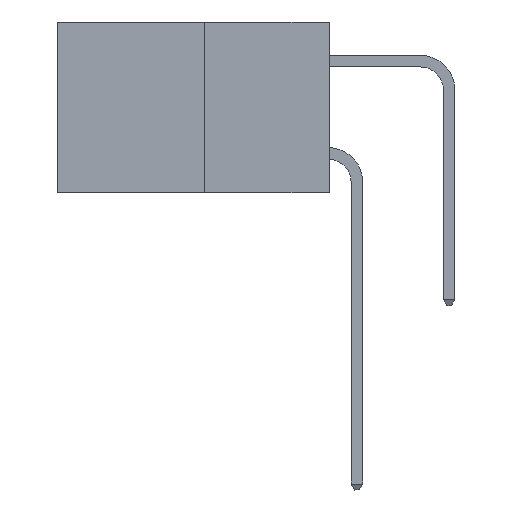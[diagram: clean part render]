
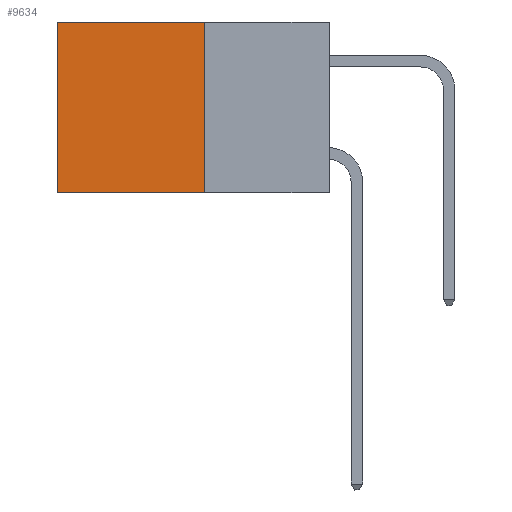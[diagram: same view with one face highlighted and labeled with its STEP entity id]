
A CAD part, left-side view. The second image highlights one B-rep face of the part: STEP entity #9634.
In plain terms, the highlighted planar face has unit normal (-1, 0, 0).
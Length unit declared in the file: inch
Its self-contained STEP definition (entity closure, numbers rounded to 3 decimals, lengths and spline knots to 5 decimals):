
#104 = DIRECTION ( 'NONE',  ( 0., 0., -1. ) ) ;
#999 = VECTOR ( 'NONE', #104, 39.37008 ) ;
#2378 = LINE ( 'NONE', #14865, #7768 ) ;
#2826 = DIRECTION ( 'NONE',  ( 0., 1., 0. ) ) ;
#3563 = VERTEX_POINT ( 'NONE', #7090 ) ;
#3830 = LINE ( 'NONE', #17312, #13896 ) ;
#3854 = DIRECTION ( 'NONE',  ( 1., 0., 0. ) ) ;
#4019 = AXIS2_PLACEMENT_3D ( 'NONE', #13872, #3854, #17817 ) ;
#5035 = ORIENTED_EDGE ( 'NONE', *, *, #22471, .F. ) ;
#5662 = VERTEX_POINT ( 'NONE', #12181 ) ;
#7090 = CARTESIAN_POINT ( 'NONE',  ( 0.277, 0.59, -0.37 ) ) ;
#7155 = CARTESIAN_POINT ( 'NONE',  ( 0.277, 0.27, 0. ) ) ;
#7768 = VECTOR ( 'NONE', #2826, 39.37008 ) ;
#9620 = DIRECTION ( 'NONE',  ( 0., 0., -1. ) ) ;
#9634 = ADVANCED_FACE ( 'NONE', ( #17830 ), #9843, .F. ) ;
#9757 = VECTOR ( 'NONE', #9620, 39.37008 ) ;
#9843 = PLANE ( 'NONE',  #4019 ) ;
#9889 = VERTEX_POINT ( 'NONE', #20337 ) ;
#10694 = EDGE_CURVE ( 'NONE', #22945, #9889, #2378, .T. ) ;
#12181 = CARTESIAN_POINT ( 'NONE',  ( 0.277, 0.27, -0.37 ) ) ;
#13182 = EDGE_LOOP ( 'NONE', ( #13650, #17788, #5035, #19282 ) ) ;
#13646 = EDGE_CURVE ( 'NONE', #5662, #3563, #3830, .T. ) ;
#13650 = ORIENTED_EDGE ( 'NONE', *, *, #19913, .T. ) ;
#13872 = CARTESIAN_POINT ( 'NONE',  ( 0.277, 0.27, -0.37 ) ) ;
#13896 = VECTOR ( 'NONE', #19266, 39.37008 ) ;
#14865 = CARTESIAN_POINT ( 'NONE',  ( 0.277, 0.27, 0. ) ) ;
#15666 = LINE ( 'NONE', #19474, #9757 ) ;
#17312 = CARTESIAN_POINT ( 'NONE',  ( 0.277, 0.27, -0.37 ) ) ;
#17788 = ORIENTED_EDGE ( 'NONE', *, *, #13646, .F. ) ;
#17817 = DIRECTION ( 'NONE',  ( 0., 0., -1. ) ) ;
#17830 = FACE_OUTER_BOUND ( 'NONE', #13182, .T. ) ;
#19266 = DIRECTION ( 'NONE',  ( 0., 1., 0. ) ) ;
#19282 = ORIENTED_EDGE ( 'NONE', *, *, #10694, .T. ) ;
#19474 = CARTESIAN_POINT ( 'NONE',  ( 0.277, 0.27, -0.37 ) ) ;
#19913 = EDGE_CURVE ( 'NONE', #9889, #3563, #22175, .T. ) ;
#20337 = CARTESIAN_POINT ( 'NONE',  ( 0.277, 0.59, 0. ) ) ;
#22175 = LINE ( 'NONE', #23888, #999 ) ;
#22471 = EDGE_CURVE ( 'NONE', #22945, #5662, #15666, .T. ) ;
#22945 = VERTEX_POINT ( 'NONE', #7155 ) ;
#23888 = CARTESIAN_POINT ( 'NONE',  ( 0.277, 0.59, -0.37 ) ) ;
